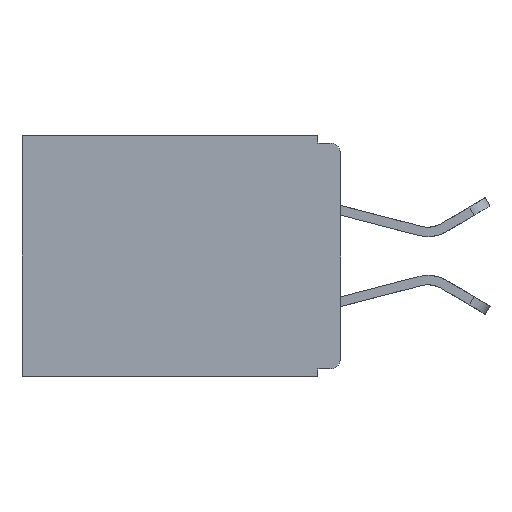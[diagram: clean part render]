
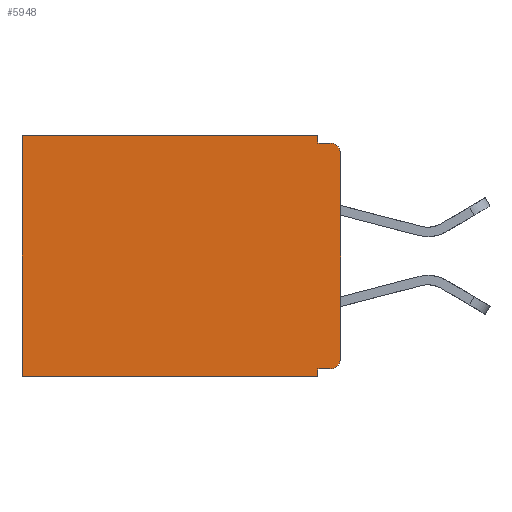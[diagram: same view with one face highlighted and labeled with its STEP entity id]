
A CAD part, left-side view. The second image highlights one B-rep face of the part: STEP entity #5948.
In plain terms, the highlighted planar face has unit normal (-1, 0, 0).
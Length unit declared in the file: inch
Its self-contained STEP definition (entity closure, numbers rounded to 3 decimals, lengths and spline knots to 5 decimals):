
#333 = VERTEX_POINT ( 'NONE', #12776 ) ;
#893 = CIRCLE ( 'NONE', #3719, 0.015 ) ;
#1217 = VERTEX_POINT ( 'NONE', #22067 ) ;
#1245 = ORIENTED_EDGE ( 'NONE', *, *, #9680, .F. ) ;
#2318 = EDGE_CURVE ( 'NONE', #12016, #22718, #19321, .T. ) ;
#3719 = AXIS2_PLACEMENT_3D ( 'NONE', #15067, #33102, #17728 ) ;
#3802 = LINE ( 'NONE', #5756, #9243 ) ;
#4268 = VECTOR ( 'NONE', #5711, 39.37008 ) ;
#4564 = LINE ( 'NONE', #29914, #17788 ) ;
#5289 = VECTOR ( 'NONE', #14250, 39.37008 ) ;
#5711 = DIRECTION ( 'NONE',  ( 0., 1., 0. ) ) ;
#5756 = CARTESIAN_POINT ( 'NONE',  ( 0.3, 0.437, -0.33 ) ) ;
#5941 = DIRECTION ( 'NONE',  ( 0., 0., -1. ) ) ;
#5948 = ADVANCED_FACE ( 'NONE', ( #18640 ), #23169, .F. ) ;
#6242 = EDGE_CURVE ( 'NONE', #20359, #14873, #3802, .T. ) ;
#6292 = ORIENTED_EDGE ( 'NONE', *, *, #22158, .F. ) ;
#7103 = EDGE_CURVE ( 'NONE', #7209, #1217, #4564, .T. ) ;
#7209 = VERTEX_POINT ( 'NONE', #32298 ) ;
#7638 = VECTOR ( 'NONE', #23918, 39.37008 ) ;
#7660 = CARTESIAN_POINT ( 'NONE',  ( 0.3, 0., 0. ) ) ;
#8069 = CARTESIAN_POINT ( 'NONE',  ( 0.3, 0., -0.33 ) ) ;
#8326 = CARTESIAN_POINT ( 'NONE',  ( 0.3, 0.031, -0.33 ) ) ;
#9243 = VECTOR ( 'NONE', #5941, 39.37008 ) ;
#9560 = AXIS2_PLACEMENT_3D ( 'NONE', #30584, #15028, #33064 ) ;
#9680 = EDGE_CURVE ( 'NONE', #1217, #24463, #28436, .T. ) ;
#9987 = ORIENTED_EDGE ( 'NONE', *, *, #6242, .T. ) ;
#10150 = CARTESIAN_POINT ( 'NONE',  ( 0.3, 0., -0.33 ) ) ;
#10487 = VECTOR ( 'NONE', #29138, 39.37008 ) ;
#11311 = LINE ( 'NONE', #26632, #4268 ) ;
#11636 = ORIENTED_EDGE ( 'NONE', *, *, #28521, .F. ) ;
#12016 = VERTEX_POINT ( 'NONE', #15659 ) ;
#12776 = CARTESIAN_POINT ( 'NONE',  ( 0.3, 0.031, -0.32 ) ) ;
#13120 = CIRCLE ( 'NONE', #9560, 0.015 ) ;
#14250 = DIRECTION ( 'NONE',  ( 0., 0., -1. ) ) ;
#14858 = VERTEX_POINT ( 'NONE', #19353 ) ;
#14873 = VERTEX_POINT ( 'NONE', #24653 ) ;
#15028 = DIRECTION ( 'NONE',  ( -1., 0., 0. ) ) ;
#15056 = CARTESIAN_POINT ( 'NONE',  ( 0.3, 0.015, -0.01 ) ) ;
#15067 = CARTESIAN_POINT ( 'NONE',  ( 0.3, 0.015, -0.025 ) ) ;
#15160 = CARTESIAN_POINT ( 'NONE',  ( 0.3, 0.031, -0.33 ) ) ;
#15659 = CARTESIAN_POINT ( 'NONE',  ( 0.3, 0., -0.025 ) ) ;
#16741 = VERTEX_POINT ( 'NONE', #15160 ) ;
#17728 = DIRECTION ( 'NONE',  ( 0., 0., -1. ) ) ;
#17788 = VECTOR ( 'NONE', #29849, 39.37008 ) ;
#18298 = LINE ( 'NONE', #8326, #10487 ) ;
#18318 = EDGE_CURVE ( 'NONE', #333, #16741, #18298, .T. ) ;
#18640 = FACE_OUTER_BOUND ( 'NONE', #19650, .T. ) ;
#19321 = LINE ( 'NONE', #8069, #5289 ) ;
#19353 = CARTESIAN_POINT ( 'NONE',  ( 0.3, 0.015, -0.32 ) ) ;
#19376 = ORIENTED_EDGE ( 'NONE', *, *, #2318, .F. ) ;
#19650 = EDGE_LOOP ( 'NONE', ( #19376, #33443, #1245, #22282, #29939, #9987, #11636, #25517, #6292, #20291 ) ) ;
#20291 = ORIENTED_EDGE ( 'NONE', *, *, #33675, .T. ) ;
#20359 = VERTEX_POINT ( 'NONE', #32440 ) ;
#20522 = CARTESIAN_POINT ( 'NONE',  ( 0.3, 0., -0.01 ) ) ;
#22067 = CARTESIAN_POINT ( 'NONE',  ( 0.3, 0.031, -0.01 ) ) ;
#22158 = EDGE_CURVE ( 'NONE', #14858, #333, #11311, .T. ) ;
#22282 = ORIENTED_EDGE ( 'NONE', *, *, #7103, .F. ) ;
#22718 = VERTEX_POINT ( 'NONE', #29289 ) ;
#23071 = DIRECTION ( 'NONE',  ( 0., 0., -1. ) ) ;
#23101 = DIRECTION ( 'NONE',  ( 1., 0., 0. ) ) ;
#23161 = CARTESIAN_POINT ( 'NONE',  ( 0.3, 0., -0.33 ) ) ;
#23169 = PLANE ( 'NONE',  #32666 ) ;
#23202 = VECTOR ( 'NONE', #28503, 39.37008 ) ;
#23812 = VECTOR ( 'NONE', #25776, 39.37008 ) ;
#23918 = DIRECTION ( 'NONE',  ( 0., -1., 0. ) ) ;
#24463 = VERTEX_POINT ( 'NONE', #15056 ) ;
#24653 = CARTESIAN_POINT ( 'NONE',  ( 0.3, 0.437, -0.33 ) ) ;
#25517 = ORIENTED_EDGE ( 'NONE', *, *, #18318, .F. ) ;
#25776 = DIRECTION ( 'NONE',  ( 0., 1., 0. ) ) ;
#26632 = CARTESIAN_POINT ( 'NONE',  ( 0.3, 0., -0.32 ) ) ;
#28436 = LINE ( 'NONE', #20522, #7638 ) ;
#28503 = DIRECTION ( 'NONE',  ( 0., 1., 0. ) ) ;
#28521 = EDGE_CURVE ( 'NONE', #16741, #14873, #29881, .T. ) ;
#29138 = DIRECTION ( 'NONE',  ( 0., 0., -1. ) ) ;
#29289 = CARTESIAN_POINT ( 'NONE',  ( 0.3, 0., -0.305 ) ) ;
#29849 = DIRECTION ( 'NONE',  ( 0., 0., -1. ) ) ;
#29881 = LINE ( 'NONE', #10150, #23812 ) ;
#29914 = CARTESIAN_POINT ( 'NONE',  ( 0.3, 0.031, 0. ) ) ;
#29939 = ORIENTED_EDGE ( 'NONE', *, *, #31969, .T. ) ;
#30584 = CARTESIAN_POINT ( 'NONE',  ( 0.3, 0.015, -0.305 ) ) ;
#30881 = LINE ( 'NONE', #7660, #23202 ) ;
#31969 = EDGE_CURVE ( 'NONE', #7209, #20359, #30881, .T. ) ;
#32298 = CARTESIAN_POINT ( 'NONE',  ( 0.3, 0.031, 0. ) ) ;
#32440 = CARTESIAN_POINT ( 'NONE',  ( 0.3, 0.437, 0. ) ) ;
#32666 = AXIS2_PLACEMENT_3D ( 'NONE', #23161, #23101, #23071 ) ;
#33062 = EDGE_CURVE ( 'NONE', #12016, #24463, #893, .T. ) ;
#33064 = DIRECTION ( 'NONE',  ( 0., 0., -1. ) ) ;
#33102 = DIRECTION ( 'NONE',  ( -1., 0., 0. ) ) ;
#33443 = ORIENTED_EDGE ( 'NONE', *, *, #33062, .T. ) ;
#33675 = EDGE_CURVE ( 'NONE', #14858, #22718, #13120, .T. ) ;
